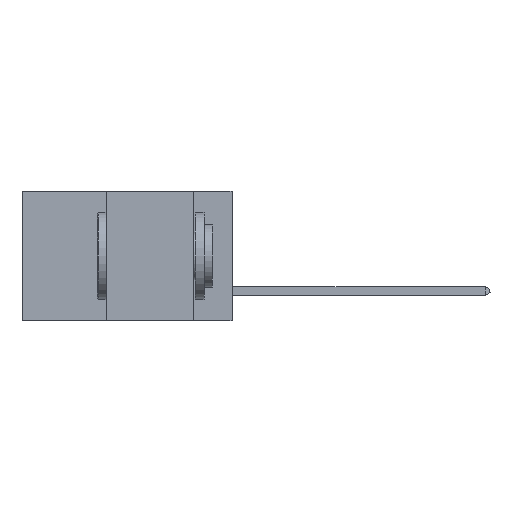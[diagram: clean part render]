
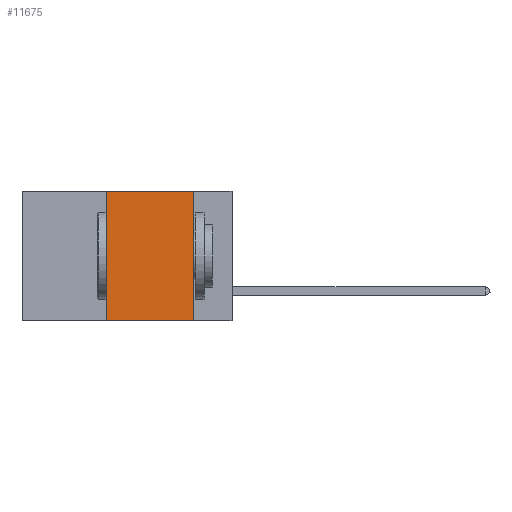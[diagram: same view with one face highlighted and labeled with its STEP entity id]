
A CAD part, left-side view. The second image highlights one B-rep face of the part: STEP entity #11675.
In plain terms, the highlighted planar face has unit normal (-1, 0, 0).
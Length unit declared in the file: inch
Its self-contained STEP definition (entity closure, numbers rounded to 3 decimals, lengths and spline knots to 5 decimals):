
#130 = ORIENTED_EDGE ( 'NONE', *, *, #7299, .F. ) ;
#153 = DIRECTION ( 'NONE',  ( 0., 0., -1. ) ) ;
#561 = DIRECTION ( 'NONE',  ( 1., 0., 0. ) ) ;
#614 = DIRECTION ( 'NONE',  ( 0., 0., -1. ) ) ;
#2904 = CARTESIAN_POINT ( 'NONE',  ( 0., 0.6, -0.37 ) ) ;
#3148 = PLANE ( 'NONE',  #13533 ) ;
#3186 = VERTEX_POINT ( 'NONE', #3728 ) ;
#3258 = LINE ( 'NONE', #3682, #14339 ) ;
#3682 = CARTESIAN_POINT ( 'NONE',  ( 0., 0.6, 0. ) ) ;
#3728 = CARTESIAN_POINT ( 'NONE',  ( 0., 0.11, -0.37 ) ) ;
#4013 = DIRECTION ( 'NONE',  ( 0., -1., 0. ) ) ;
#4354 = EDGE_CURVE ( 'NONE', #15854, #3186, #15475, .T. ) ;
#5208 = EDGE_LOOP ( 'NONE', ( #10578, #11614, #130, #11723 ) ) ;
#5893 = VECTOR ( 'NONE', #4013, 39.37008 ) ;
#5984 = VERTEX_POINT ( 'NONE', #13072 ) ;
#6717 = LINE ( 'NONE', #7705, #14135 ) ;
#7299 = EDGE_CURVE ( 'NONE', #15854, #5984, #10922, .T. ) ;
#7705 = CARTESIAN_POINT ( 'NONE',  ( 0., 0.11, 0. ) ) ;
#9032 = EDGE_CURVE ( 'NONE', #9888, #3186, #6717, .T. ) ;
#9740 = VECTOR ( 'NONE', #15459, 39.37008 ) ;
#9874 = FACE_OUTER_BOUND ( 'NONE', #5208, .T. ) ;
#9888 = VERTEX_POINT ( 'NONE', #13568 ) ;
#10578 = ORIENTED_EDGE ( 'NONE', *, *, #9032, .F. ) ;
#10922 = LINE ( 'NONE', #15635, #9740 ) ;
#10928 = EDGE_CURVE ( 'NONE', #5984, #9888, #3258, .T. ) ;
#11614 = ORIENTED_EDGE ( 'NONE', *, *, #10928, .F. ) ;
#11675 = ADVANCED_FACE ( 'NONE', ( #9874 ), #3148, .F. ) ;
#11723 = ORIENTED_EDGE ( 'NONE', *, *, #4354, .T. ) ;
#12432 = DIRECTION ( 'NONE',  ( 0., -1., 0. ) ) ;
#13072 = CARTESIAN_POINT ( 'NONE',  ( 0., 0.36, 0. ) ) ;
#13533 = AXIS2_PLACEMENT_3D ( 'NONE', #15559, #561, #614 ) ;
#13568 = CARTESIAN_POINT ( 'NONE',  ( 0., 0.11, 0. ) ) ;
#14135 = VECTOR ( 'NONE', #153, 39.37008 ) ;
#14339 = VECTOR ( 'NONE', #12432, 39.37008 ) ;
#14594 = CARTESIAN_POINT ( 'NONE',  ( 0., 0.36, -0.37 ) ) ;
#15459 = DIRECTION ( 'NONE',  ( 0., 0., 1. ) ) ;
#15475 = LINE ( 'NONE', #2904, #5893 ) ;
#15559 = CARTESIAN_POINT ( 'NONE',  ( 0., 0.6, 0. ) ) ;
#15635 = CARTESIAN_POINT ( 'NONE',  ( 0., 0.36, 0. ) ) ;
#15854 = VERTEX_POINT ( 'NONE', #14594 ) ;
